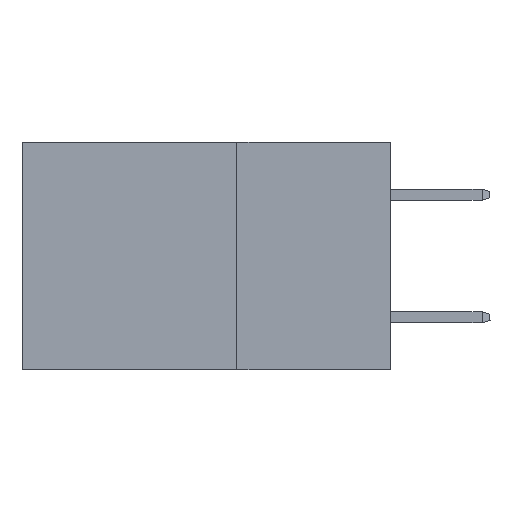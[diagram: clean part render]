
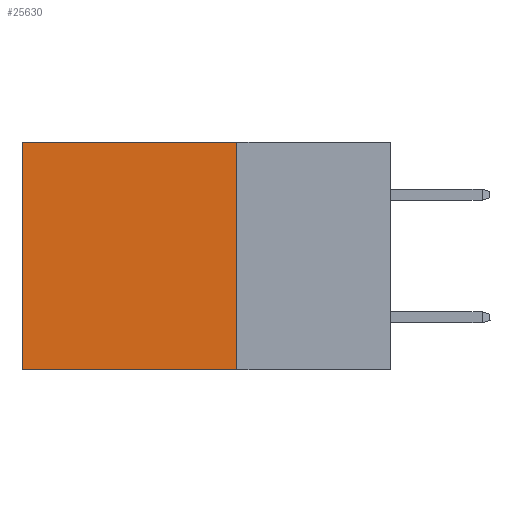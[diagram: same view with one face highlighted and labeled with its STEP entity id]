
A CAD part, left-side view. The second image highlights one B-rep face of the part: STEP entity #25630.
In plain terms, the highlighted planar face has unit normal (-1, 0, 0).
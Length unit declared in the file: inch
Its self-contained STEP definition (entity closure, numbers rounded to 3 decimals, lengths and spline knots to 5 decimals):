
#576 = AXIS2_PLACEMENT_3D ( 'NONE', #25818, #11621, #16414 ) ;
#843 = EDGE_CURVE ( 'NONE', #12744, #3118, #3568, .T. ) ;
#1916 = CARTESIAN_POINT ( 'NONE',  ( 0.2875, 0.6, -0.37 ) ) ;
#2481 = VECTOR ( 'NONE', #14972, 39.37008 ) ;
#3118 = VERTEX_POINT ( 'NONE', #1916 ) ;
#3441 = CARTESIAN_POINT ( 'NONE',  ( 0.2875, 0.6, 0. ) ) ;
#3568 = LINE ( 'NONE', #5474, #21190 ) ;
#4699 = ORIENTED_EDGE ( 'NONE', *, *, #23699, .T. ) ;
#4834 = ORIENTED_EDGE ( 'NONE', *, *, #843, .F. ) ;
#5474 = CARTESIAN_POINT ( 'NONE',  ( 0.2875, 0.25, -0.37 ) ) ;
#6647 = VECTOR ( 'NONE', #15397, 39.37008 ) ;
#7671 = DIRECTION ( 'NONE',  ( 0., 1., 0. ) ) ;
#8731 = CARTESIAN_POINT ( 'NONE',  ( 0.2875, 0.25, 0. ) ) ;
#9685 = PLANE ( 'NONE',  #576 ) ;
#9853 = FACE_OUTER_BOUND ( 'NONE', #29073, .T. ) ;
#11299 = LINE ( 'NONE', #8731, #14884 ) ;
#11621 = DIRECTION ( 'NONE',  ( 1., 0., 0. ) ) ;
#12744 = VERTEX_POINT ( 'NONE', #29399 ) ;
#13457 = VERTEX_POINT ( 'NONE', #20206 ) ;
#14884 = VECTOR ( 'NONE', #22657, 39.37008 ) ;
#14972 = DIRECTION ( 'NONE',  ( 0., 0., -1. ) ) ;
#15397 = DIRECTION ( 'NONE',  ( 0., 0., -1. ) ) ;
#16414 = DIRECTION ( 'NONE',  ( 0., 0., -1. ) ) ;
#17034 = VERTEX_POINT ( 'NONE', #18604 ) ;
#17193 = LINE ( 'NONE', #3441, #2481 ) ;
#18604 = CARTESIAN_POINT ( 'NONE',  ( 0.2875, 0.25, 0. ) ) ;
#20206 = CARTESIAN_POINT ( 'NONE',  ( 0.2875, 0.6, 0. ) ) ;
#20542 = ORIENTED_EDGE ( 'NONE', *, *, #26798, .T. ) ;
#21190 = VECTOR ( 'NONE', #7671, 39.37008 ) ;
#22657 = DIRECTION ( 'NONE',  ( 0., 1., 0. ) ) ;
#23064 = ORIENTED_EDGE ( 'NONE', *, *, #26652, .F. ) ;
#23699 = EDGE_CURVE ( 'NONE', #13457, #3118, #17193, .T. ) ;
#24292 = LINE ( 'NONE', #26885, #6647 ) ;
#25630 = ADVANCED_FACE ( 'NONE', ( #9853 ), #9685, .F. ) ;
#25818 = CARTESIAN_POINT ( 'NONE',  ( 0.2875, 0.25, 0. ) ) ;
#26652 = EDGE_CURVE ( 'NONE', #17034, #12744, #24292, .T. ) ;
#26798 = EDGE_CURVE ( 'NONE', #17034, #13457, #11299, .T. ) ;
#26885 = CARTESIAN_POINT ( 'NONE',  ( 0.2875, 0.25, 0. ) ) ;
#29073 = EDGE_LOOP ( 'NONE', ( #4699, #4834, #23064, #20542 ) ) ;
#29399 = CARTESIAN_POINT ( 'NONE',  ( 0.2875, 0.25, -0.37 ) ) ;
